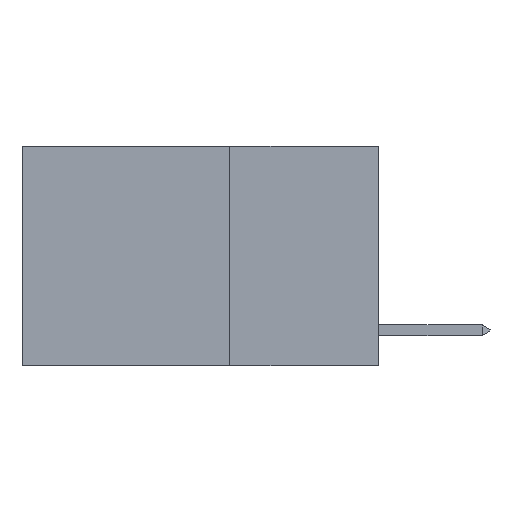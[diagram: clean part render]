
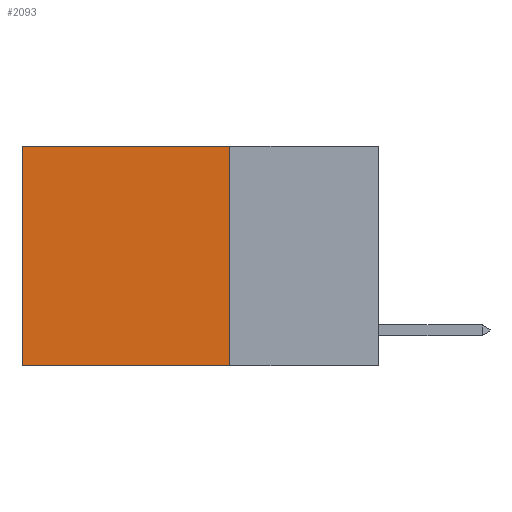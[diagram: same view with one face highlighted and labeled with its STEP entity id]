
A CAD part, left-side view. The second image highlights one B-rep face of the part: STEP entity #2093.
In plain terms, the highlighted planar face has unit normal (-1, 0, 0).
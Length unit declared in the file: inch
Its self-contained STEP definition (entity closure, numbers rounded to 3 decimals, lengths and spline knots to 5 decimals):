
#18 = CARTESIAN_POINT ( 'NONE',  ( 0.2625, 0.25, -0.37 ) ) ;
#217 = LINE ( 'NONE', #3917, #6490 ) ;
#475 = CARTESIAN_POINT ( 'NONE',  ( 0.2625, 0.25, 0. ) ) ;
#500 = VECTOR ( 'NONE', #4161, 39.37008 ) ;
#542 = LINE ( 'NONE', #5048, #500 ) ;
#985 = EDGE_CURVE ( 'NONE', #4136, #5451, #2303, .T. ) ;
#1223 = FACE_OUTER_BOUND ( 'NONE', #4708, .T. ) ;
#1608 = DIRECTION ( 'NONE',  ( 0., 1., 0. ) ) ;
#1879 = VERTEX_POINT ( 'NONE', #4020 ) ;
#2093 = ADVANCED_FACE ( 'NONE', ( #1223 ), #9367, .F. ) ;
#2175 = VERTEX_POINT ( 'NONE', #6353 ) ;
#2291 = VECTOR ( 'NONE', #3903, 39.37008 ) ;
#2303 = LINE ( 'NONE', #4099, #2291 ) ;
#2637 = ORIENTED_EDGE ( 'NONE', *, *, #985, .F. ) ;
#3903 = DIRECTION ( 'NONE',  ( 0., 0., -1. ) ) ;
#3917 = CARTESIAN_POINT ( 'NONE',  ( 0.2625, 0.25, 0. ) ) ;
#4020 = CARTESIAN_POINT ( 'NONE',  ( 0.2625, 0.6, -0.37 ) ) ;
#4099 = CARTESIAN_POINT ( 'NONE',  ( 0.2625, 0.25, 0. ) ) ;
#4136 = VERTEX_POINT ( 'NONE', #475 ) ;
#4161 = DIRECTION ( 'NONE',  ( 0., 1., 0. ) ) ;
#4366 = EDGE_CURVE ( 'NONE', #2175, #1879, #5180, .T. ) ;
#4708 = EDGE_LOOP ( 'NONE', ( #7578, #8993, #2637, #5616 ) ) ;
#4894 = CARTESIAN_POINT ( 'NONE',  ( 0.2625, 0.6, 0. ) ) ;
#4913 = DIRECTION ( 'NONE',  ( 0., 0., -1. ) ) ;
#5048 = CARTESIAN_POINT ( 'NONE',  ( 0.2625, 0.25, -0.37 ) ) ;
#5093 = VECTOR ( 'NONE', #4913, 39.37008 ) ;
#5180 = LINE ( 'NONE', #4894, #5093 ) ;
#5451 = VERTEX_POINT ( 'NONE', #18 ) ;
#5616 = ORIENTED_EDGE ( 'NONE', *, *, #9055, .T. ) ;
#5686 = AXIS2_PLACEMENT_3D ( 'NONE', #9010, #8954, #8933 ) ;
#6353 = CARTESIAN_POINT ( 'NONE',  ( 0.2625, 0.6, 0. ) ) ;
#6490 = VECTOR ( 'NONE', #1608, 39.37008 ) ;
#7578 = ORIENTED_EDGE ( 'NONE', *, *, #4366, .T. ) ;
#7635 = EDGE_CURVE ( 'NONE', #5451, #1879, #542, .T. ) ;
#8933 = DIRECTION ( 'NONE',  ( 0., 0., -1. ) ) ;
#8954 = DIRECTION ( 'NONE',  ( 1., 0., 0. ) ) ;
#8993 = ORIENTED_EDGE ( 'NONE', *, *, #7635, .F. ) ;
#9010 = CARTESIAN_POINT ( 'NONE',  ( 0.2625, 0.25, 0. ) ) ;
#9055 = EDGE_CURVE ( 'NONE', #4136, #2175, #217, .T. ) ;
#9367 = PLANE ( 'NONE',  #5686 ) ;
